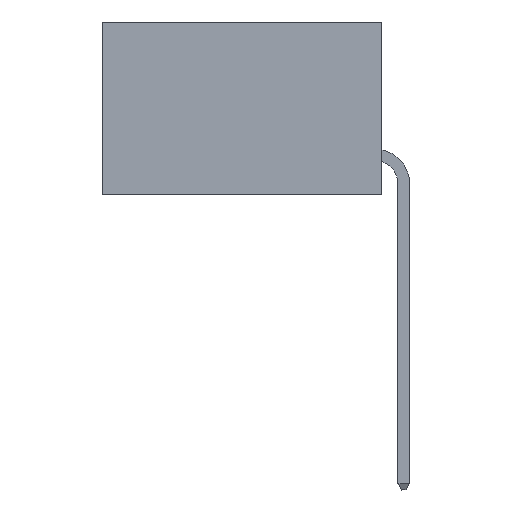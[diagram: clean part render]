
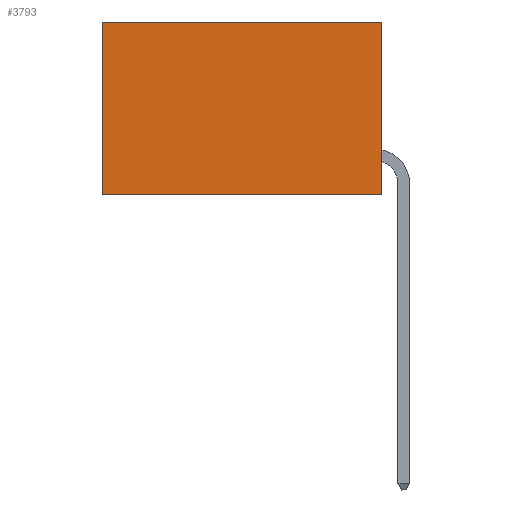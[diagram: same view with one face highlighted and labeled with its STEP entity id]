
A CAD part, left-side view. The second image highlights one B-rep face of the part: STEP entity #3793.
In plain terms, the highlighted planar face has unit normal (-1, 0, 0).
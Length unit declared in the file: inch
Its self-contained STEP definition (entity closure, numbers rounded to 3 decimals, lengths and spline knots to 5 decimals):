
#1010 = VECTOR ( 'NONE', #12719, 39.37008 ) ;
#1249 = CARTESIAN_POINT ( 'NONE',  ( 0.2875, 0., -0.37 ) ) ;
#1755 = VERTEX_POINT ( 'NONE', #1249 ) ;
#1959 = CARTESIAN_POINT ( 'NONE',  ( 0.2875, 0.6, 0. ) ) ;
#2043 = CARTESIAN_POINT ( 'NONE',  ( 0.2875, 0.6, 0. ) ) ;
#3793 = ADVANCED_FACE ( 'NONE', ( #5919 ), #5558, .F. ) ;
#4031 = DIRECTION ( 'NONE',  ( 0., 0., -1. ) ) ;
#4036 = CARTESIAN_POINT ( 'NONE',  ( 0.2875, 0., 0. ) ) ;
#5558 = PLANE ( 'NONE',  #7899 ) ;
#5703 = CARTESIAN_POINT ( 'NONE',  ( 0.2875, 0.6, -0.37 ) ) ;
#5919 = FACE_OUTER_BOUND ( 'NONE', #21940, .T. ) ;
#5951 = CARTESIAN_POINT ( 'NONE',  ( 0.2875, 0., 0. ) ) ;
#6059 = ORIENTED_EDGE ( 'NONE', *, *, #25669, .F. ) ;
#6325 = EDGE_CURVE ( 'NONE', #1755, #10059, #19391, .T. ) ;
#6700 = VECTOR ( 'NONE', #21097, 39.37008 ) ;
#7899 = AXIS2_PLACEMENT_3D ( 'NONE', #27691, #23072, #16660 ) ;
#8740 = VERTEX_POINT ( 'NONE', #2043 ) ;
#8993 = ORIENTED_EDGE ( 'NONE', *, *, #20510, .T. ) ;
#9639 = CARTESIAN_POINT ( 'NONE',  ( 0.2875, 0., -0.37 ) ) ;
#10059 = VERTEX_POINT ( 'NONE', #5703 ) ;
#11134 = VECTOR ( 'NONE', #19366, 39.37008 ) ;
#11878 = VECTOR ( 'NONE', #4031, 39.37008 ) ;
#12719 = DIRECTION ( 'NONE',  ( 0., 0., -1. ) ) ;
#13157 = LINE ( 'NONE', #23566, #11134 ) ;
#15250 = VERTEX_POINT ( 'NONE', #5951 ) ;
#16660 = DIRECTION ( 'NONE',  ( 0., 0., -1. ) ) ;
#17685 = LINE ( 'NONE', #1959, #11878 ) ;
#18946 = ORIENTED_EDGE ( 'NONE', *, *, #6325, .F. ) ;
#19366 = DIRECTION ( 'NONE',  ( 0., 1., 0. ) ) ;
#19391 = LINE ( 'NONE', #9639, #6700 ) ;
#20510 = EDGE_CURVE ( 'NONE', #8740, #10059, #17685, .T. ) ;
#21097 = DIRECTION ( 'NONE',  ( 0., 1., 0. ) ) ;
#21940 = EDGE_LOOP ( 'NONE', ( #8993, #18946, #6059, #26352 ) ) ;
#23072 = DIRECTION ( 'NONE',  ( 1., 0., 0. ) ) ;
#23566 = CARTESIAN_POINT ( 'NONE',  ( 0.2875, 0., 0. ) ) ;
#25669 = EDGE_CURVE ( 'NONE', #15250, #1755, #25967, .T. ) ;
#25967 = LINE ( 'NONE', #4036, #1010 ) ;
#26352 = ORIENTED_EDGE ( 'NONE', *, *, #27537, .T. ) ;
#27537 = EDGE_CURVE ( 'NONE', #15250, #8740, #13157, .T. ) ;
#27691 = CARTESIAN_POINT ( 'NONE',  ( 0.2875, 0., 0. ) ) ;
